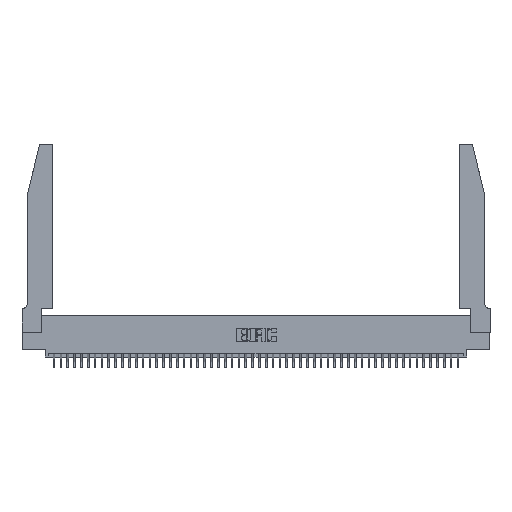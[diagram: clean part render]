
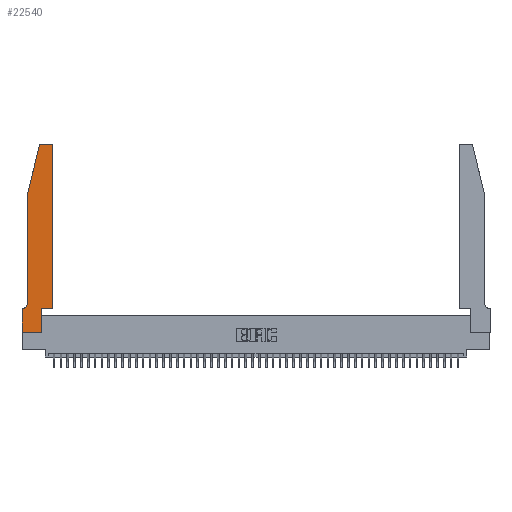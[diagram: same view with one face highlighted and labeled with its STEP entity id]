
A CAD part, top view. The second image highlights one B-rep face of the part: STEP entity #22540.
In plain terms, the highlighted planar face has unit normal (0, 0, 1).
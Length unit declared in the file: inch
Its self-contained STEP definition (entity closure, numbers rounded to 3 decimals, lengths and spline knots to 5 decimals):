
#1010 = DIRECTION ( 'NONE',  ( -0.239, -0.971, 0. ) ) ;
#1284 = CARTESIAN_POINT ( 'NONE',  ( 0., 0.35, 0.37 ) ) ;
#1560 = CARTESIAN_POINT ( 'NONE',  ( 0.2605, 2.75, 0.37 ) ) ;
#3025 = LINE ( 'NONE', #29322, #23590 ) ;
#3066 = ORIENTED_EDGE ( 'NONE', *, *, #36156, .T. ) ;
#4012 = EDGE_CURVE ( 'NONE', #45547, #15766, #19084, .T. ) ;
#5542 = ORIENTED_EDGE ( 'NONE', *, *, #4012, .T. ) ;
#5755 = CARTESIAN_POINT ( 'NONE',  ( 0.2865, 0.35, 0.37 ) ) ;
#6256 = EDGE_LOOP ( 'NONE', ( #46511, #48332, #11999, #29548, #49322, #44186, #16314, #19970, #46709, #5542, #21426, #3066 ) ) ;
#7332 = CARTESIAN_POINT ( 'NONE',  ( 0.0755, 2., 0.37 ) ) ;
#7486 = VECTOR ( 'NONE', #47921, 39.37008 ) ;
#8259 = CIRCLE ( 'NONE', #38768, 0.07 ) ;
#9798 = DIRECTION ( 'NONE',  ( 0., 0., -1. ) ) ;
#10397 = EDGE_CURVE ( 'NONE', #33450, #39312, #36575, .T. ) ;
#11029 = LINE ( 'NONE', #1560, #20112 ) ;
#11109 = LINE ( 'NONE', #39606, #21397 ) ;
#11148 = VERTEX_POINT ( 'NONE', #38656 ) ;
#11999 = ORIENTED_EDGE ( 'NONE', *, *, #30556, .T. ) ;
#12119 = CIRCLE ( 'NONE', #38200, 0.03 ) ;
#12323 = CIRCLE ( 'NONE', #39741, 0.03 ) ;
#13100 = CARTESIAN_POINT ( 'NONE',  ( 0.4205, 2.75, 0.37 ) ) ;
#13631 = CARTESIAN_POINT ( 'NONE',  ( 0., 0., 0.37 ) ) ;
#14013 = CARTESIAN_POINT ( 'NONE',  ( 0.284, 2.72, 0.37 ) ) ;
#14027 = VERTEX_POINT ( 'NONE', #26918 ) ;
#15766 = VERTEX_POINT ( 'NONE', #34025 ) ;
#15999 = EDGE_CURVE ( 'NONE', #32039, #11148, #23518, .T. ) ;
#16314 = ORIENTED_EDGE ( 'NONE', *, *, #15999, .T. ) ;
#16352 = LINE ( 'NONE', #5755, #43253 ) ;
#16372 = DIRECTION ( 'NONE',  ( 0., 0., 1. ) ) ;
#16789 = VERTEX_POINT ( 'NONE', #13100 ) ;
#16836 = DIRECTION ( 'NONE',  ( 1., 0., 0. ) ) ;
#17403 = CARTESIAN_POINT ( 'NONE',  ( 0., 0.35, 0.37 ) ) ;
#17898 = DIRECTION ( 'NONE',  ( 1., 0., 0. ) ) ;
#18961 = VERTEX_POINT ( 'NONE', #21209 ) ;
#19084 = LINE ( 'NONE', #39771, #30491 ) ;
#19928 = DIRECTION ( 'NONE',  ( 0., -1., 0. ) ) ;
#19970 = ORIENTED_EDGE ( 'NONE', *, *, #34452, .T. ) ;
#20112 = VECTOR ( 'NONE', #24748, 39.37008 ) ;
#21209 = CARTESIAN_POINT ( 'NONE',  ( 0.0055, 0.35, 0.37 ) ) ;
#21224 = DIRECTION ( 'NONE',  ( 0., 1., 0. ) ) ;
#21267 = DIRECTION ( 'NONE',  ( 1., 0., 0. ) ) ;
#21397 = VECTOR ( 'NONE', #35794, 39.37008 ) ;
#21426 = ORIENTED_EDGE ( 'NONE', *, *, #47027, .T. ) ;
#22340 = DIRECTION ( 'NONE',  ( 0., -1., 0. ) ) ;
#22540 = ADVANCED_FACE ( 'NONE', ( #47813 ), #28815, .T. ) ;
#22559 = EDGE_CURVE ( 'NONE', #39312, #18961, #8259, .T. ) ;
#23518 = LINE ( 'NONE', #31478, #32484 ) ;
#23590 = VECTOR ( 'NONE', #33169, 39.37008 ) ;
#24748 = DIRECTION ( 'NONE',  ( -1., 0., 0. ) ) ;
#25203 = VECTOR ( 'NONE', #22340, 39.37008 ) ;
#26220 = CARTESIAN_POINT ( 'NONE',  ( 0.0755, 2., 0.37 ) ) ;
#26918 = CARTESIAN_POINT ( 'NONE',  ( 0.2865, 0., 0.37 ) ) ;
#26974 = VERTEX_POINT ( 'NONE', #38034 ) ;
#27104 = CARTESIAN_POINT ( 'NONE',  ( 0.0755, 0.42, 0.37 ) ) ;
#28815 = PLANE ( 'NONE',  #41299 ) ;
#29322 = CARTESIAN_POINT ( 'NONE',  ( 0.0755, 0.35, 0.37 ) ) ;
#29548 = ORIENTED_EDGE ( 'NONE', *, *, #10397, .T. ) ;
#30491 = VECTOR ( 'NONE', #16836, 39.37008 ) ;
#30556 = EDGE_CURVE ( 'NONE', #43066, #33450, #42645, .T. ) ;
#30693 = CARTESIAN_POINT ( 'NONE',  ( 0.2865, 0.35, 0.37 ) ) ;
#31478 = CARTESIAN_POINT ( 'NONE',  ( 0., 0., 0.37 ) ) ;
#32039 = VERTEX_POINT ( 'NONE', #1284 ) ;
#32484 = VECTOR ( 'NONE', #19928, 39.37008 ) ;
#32528 = VECTOR ( 'NONE', #1010, 39.37008 ) ;
#32833 = CARTESIAN_POINT ( 'NONE',  ( 0.0055, 0.42, 0.37 ) ) ;
#33169 = DIRECTION ( 'NONE',  ( -1., 0., 0. ) ) ;
#33450 = VERTEX_POINT ( 'NONE', #7332 ) ;
#34025 = CARTESIAN_POINT ( 'NONE',  ( 0.4505, 0.35, 0.37 ) ) ;
#34452 = EDGE_CURVE ( 'NONE', #11148, #14027, #36924, .T. ) ;
#35794 = DIRECTION ( 'NONE',  ( 0., 1., 0. ) ) ;
#36156 = EDGE_CURVE ( 'NONE', #26974, #16789, #12119, .T. ) ;
#36234 = CARTESIAN_POINT ( 'NONE',  ( 0.25487, 2.72718, 0.37 ) ) ;
#36285 = EDGE_CURVE ( 'NONE', #14027, #45547, #16352, .T. ) ;
#36575 = LINE ( 'NONE', #26220, #25203 ) ;
#36670 = DIRECTION ( 'NONE',  ( -1., 0., 0. ) ) ;
#36924 = LINE ( 'NONE', #13631, #7486 ) ;
#38034 = CARTESIAN_POINT ( 'NONE',  ( 0.4505, 2.72, 0.37 ) ) ;
#38200 = AXIS2_PLACEMENT_3D ( 'NONE', #39298, #16372, #43110 ) ;
#38656 = CARTESIAN_POINT ( 'NONE',  ( 0., 0., 0.37 ) ) ;
#38687 = VERTEX_POINT ( 'NONE', #42468 ) ;
#38768 = AXIS2_PLACEMENT_3D ( 'NONE', #32833, #9798, #36670 ) ;
#39298 = CARTESIAN_POINT ( 'NONE',  ( 0.4205, 2.72, 0.37 ) ) ;
#39312 = VERTEX_POINT ( 'NONE', #27104 ) ;
#39606 = CARTESIAN_POINT ( 'NONE',  ( 0.4505, 0.35, 0.37 ) ) ;
#39741 = AXIS2_PLACEMENT_3D ( 'NONE', #14013, #40794, #17898 ) ;
#39771 = CARTESIAN_POINT ( 'NONE',  ( 0.4505, 0.35, 0.37 ) ) ;
#40056 = EDGE_CURVE ( 'NONE', #38687, #43066, #12323, .T. ) ;
#40608 = EDGE_CURVE ( 'NONE', #16789, #38687, #11029, .T. ) ;
#40794 = DIRECTION ( 'NONE',  ( 0., 0., 1. ) ) ;
#41299 = AXIS2_PLACEMENT_3D ( 'NONE', #17403, #44148, #21267 ) ;
#41898 = EDGE_CURVE ( 'NONE', #18961, #32039, #3025, .T. ) ;
#42468 = CARTESIAN_POINT ( 'NONE',  ( 0.284, 2.75, 0.37 ) ) ;
#42645 = LINE ( 'NONE', #47086, #32528 ) ;
#43066 = VERTEX_POINT ( 'NONE', #36234 ) ;
#43110 = DIRECTION ( 'NONE',  ( 1., 0., 0. ) ) ;
#43253 = VECTOR ( 'NONE', #21224, 39.37008 ) ;
#44148 = DIRECTION ( 'NONE',  ( 0., 0., 1. ) ) ;
#44186 = ORIENTED_EDGE ( 'NONE', *, *, #41898, .T. ) ;
#45547 = VERTEX_POINT ( 'NONE', #30693 ) ;
#46511 = ORIENTED_EDGE ( 'NONE', *, *, #40608, .T. ) ;
#46709 = ORIENTED_EDGE ( 'NONE', *, *, #36285, .T. ) ;
#47027 = EDGE_CURVE ( 'NONE', #15766, #26974, #11109, .T. ) ;
#47086 = CARTESIAN_POINT ( 'NONE',  ( 0.0755, 2., 0.37 ) ) ;
#47813 = FACE_OUTER_BOUND ( 'NONE', #6256, .T. ) ;
#47921 = DIRECTION ( 'NONE',  ( 1., 0., 0. ) ) ;
#48332 = ORIENTED_EDGE ( 'NONE', *, *, #40056, .T. ) ;
#49322 = ORIENTED_EDGE ( 'NONE', *, *, #22559, .T. ) ;
